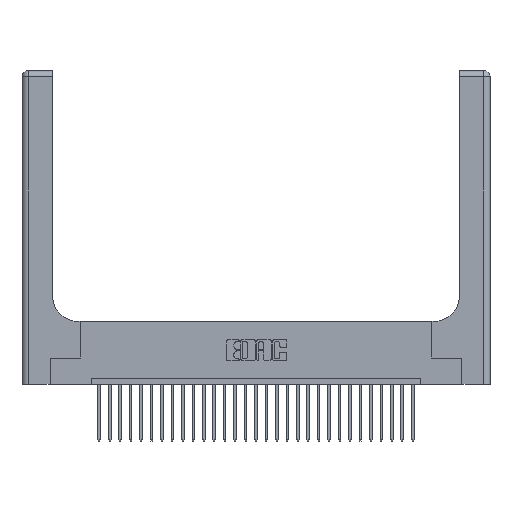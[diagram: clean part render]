
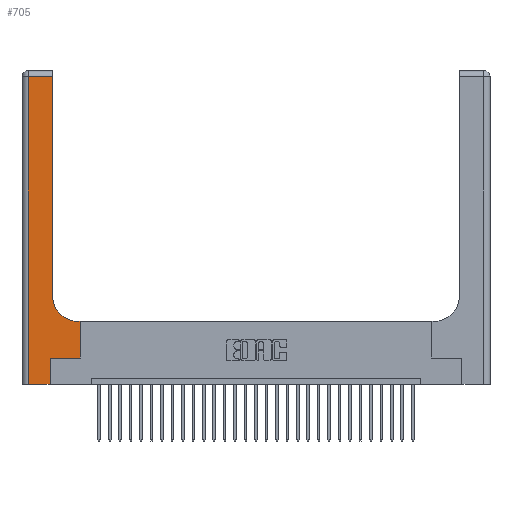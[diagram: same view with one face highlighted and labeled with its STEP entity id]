
A CAD part, top view. The second image highlights one B-rep face of the part: STEP entity #705.
In plain terms, the highlighted planar face has unit normal (0, 0, 1).
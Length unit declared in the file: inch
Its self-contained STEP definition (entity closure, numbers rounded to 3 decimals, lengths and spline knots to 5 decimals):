
#705 = ADVANCED_FACE ( 'NONE', ( #14279 ), #8738, .F. ) ;
#729 = VERTEX_POINT ( 'NONE', #22500 ) ;
#1054 = CARTESIAN_POINT ( 'NONE',  ( 0.2915, 3., 0.37 ) ) ;
#1261 = DIRECTION ( 'NONE',  ( -1., 0., 0. ) ) ;
#1467 = CARTESIAN_POINT ( 'NONE',  ( 0.06, 0., 0.37 ) ) ;
#1710 = DIRECTION ( 'NONE',  ( 0., 1., 0. ) ) ;
#3113 = CARTESIAN_POINT ( 'NONE',  ( 0.5415, 0.6, 0.37 ) ) ;
#3358 = DIRECTION ( 'NONE',  ( 0., 1., 0. ) ) ;
#3384 = ORIENTED_EDGE ( 'NONE', *, *, #9870, .T. ) ;
#3589 = VERTEX_POINT ( 'NONE', #6046 ) ;
#3943 = EDGE_CURVE ( 'NONE', #29154, #3589, #11376, .T. ) ;
#4304 = CARTESIAN_POINT ( 'NONE',  ( 0., 0., 0.37 ) ) ;
#4656 = LINE ( 'NONE', #16124, #25334 ) ;
#4949 = DIRECTION ( 'NONE',  ( 0., -1., 0. ) ) ;
#5971 = LINE ( 'NONE', #13246, #21901 ) ;
#6046 = CARTESIAN_POINT ( 'NONE',  ( 0.2915, 0.85, 0.37 ) ) ;
#6088 = VECTOR ( 'NONE', #1261, 39.37008 ) ;
#6278 = CARTESIAN_POINT ( 'NONE',  ( 0.06, 2.94, 0.37 ) ) ;
#6404 = DIRECTION ( 'NONE',  ( -1., 0., 0. ) ) ;
#7269 = VECTOR ( 'NONE', #21308, 39.37008 ) ;
#7671 = EDGE_CURVE ( 'NONE', #729, #29154, #24580, .T. ) ;
#8009 = LINE ( 'NONE', #14727, #7269 ) ;
#8738 = PLANE ( 'NONE',  #15357 ) ;
#9033 = EDGE_CURVE ( 'NONE', #27274, #27292, #15082, .T. ) ;
#9227 = DIRECTION ( 'NONE',  ( 1., 0., 0. ) ) ;
#9336 = AXIS2_PLACEMENT_3D ( 'NONE', #28037, #25803, #16454 ) ;
#9870 = EDGE_CURVE ( 'NONE', #26841, #729, #5971, .T. ) ;
#9909 = LINE ( 'NONE', #10806, #21162 ) ;
#10383 = EDGE_CURVE ( 'NONE', #23092, #25171, #9909, .T. ) ;
#10715 = ORIENTED_EDGE ( 'NONE', *, *, #24664, .T. ) ;
#10806 = CARTESIAN_POINT ( 'NONE',  ( 0., 2.94, 0.37 ) ) ;
#11376 = CIRCLE ( 'NONE', #9336, 0.25 ) ;
#13116 = LINE ( 'NONE', #1054, #28707 ) ;
#13246 = CARTESIAN_POINT ( 'NONE',  ( 0.5585, 0.25, 0.37 ) ) ;
#13258 = VECTOR ( 'NONE', #27331, 39.37008 ) ;
#13405 = CARTESIAN_POINT ( 'NONE',  ( 0., 3., 0.37 ) ) ;
#14279 = FACE_OUTER_BOUND ( 'NONE', #23038, .T. ) ;
#14501 = VECTOR ( 'NONE', #4949, 39.37008 ) ;
#14727 = CARTESIAN_POINT ( 'NONE',  ( 0.269, 0., 0.37 ) ) ;
#15082 = LINE ( 'NONE', #4304, #13258 ) ;
#15357 = AXIS2_PLACEMENT_3D ( 'NONE', #13405, #22401, #6404 ) ;
#15387 = ORIENTED_EDGE ( 'NONE', *, *, #21820, .T. ) ;
#15731 = ORIENTED_EDGE ( 'NONE', *, *, #23137, .T. ) ;
#16124 = CARTESIAN_POINT ( 'NONE',  ( 0.269, 0.25, 0.37 ) ) ;
#16454 = DIRECTION ( 'NONE',  ( 1., 0., 0. ) ) ;
#17380 = LINE ( 'NONE', #18813, #14501 ) ;
#17891 = DIRECTION ( 'NONE',  ( -1., 0., 0. ) ) ;
#17908 = ORIENTED_EDGE ( 'NONE', *, *, #3943, .T. ) ;
#18813 = CARTESIAN_POINT ( 'NONE',  ( 0.06, 3., 0.37 ) ) ;
#18849 = CARTESIAN_POINT ( 'NONE',  ( 0.2915, 2.94, 0.37 ) ) ;
#18965 = ORIENTED_EDGE ( 'NONE', *, *, #9033, .T. ) ;
#19149 = ORIENTED_EDGE ( 'NONE', *, *, #10383, .T. ) ;
#19775 = CARTESIAN_POINT ( 'NONE',  ( 0.2915, 0.6, 0.37 ) ) ;
#19794 = CARTESIAN_POINT ( 'NONE',  ( 0.269, 0.25, 0.37 ) ) ;
#19985 = EDGE_CURVE ( 'NONE', #27292, #26231, #8009, .T. ) ;
#21162 = VECTOR ( 'NONE', #17891, 39.37008 ) ;
#21308 = DIRECTION ( 'NONE',  ( 0., 1., 0. ) ) ;
#21820 = EDGE_CURVE ( 'NONE', #25171, #27274, #17380, .T. ) ;
#21901 = VECTOR ( 'NONE', #1710, 39.37008 ) ;
#22401 = DIRECTION ( 'NONE',  ( 0., 0., -1. ) ) ;
#22500 = CARTESIAN_POINT ( 'NONE',  ( 0.5585, 0.6, 0.37 ) ) ;
#23038 = EDGE_LOOP ( 'NONE', ( #15731, #19149, #15387, #18965, #27157, #10715, #3384, #26258, #17908 ) ) ;
#23092 = VERTEX_POINT ( 'NONE', #18849 ) ;
#23137 = EDGE_CURVE ( 'NONE', #3589, #23092, #13116, .T. ) ;
#24580 = LINE ( 'NONE', #19775, #6088 ) ;
#24664 = EDGE_CURVE ( 'NONE', #26231, #26841, #4656, .T. ) ;
#25171 = VERTEX_POINT ( 'NONE', #6278 ) ;
#25334 = VECTOR ( 'NONE', #9227, 39.37008 ) ;
#25803 = DIRECTION ( 'NONE',  ( 0., 0., -1. ) ) ;
#26231 = VERTEX_POINT ( 'NONE', #19794 ) ;
#26258 = ORIENTED_EDGE ( 'NONE', *, *, #7671, .T. ) ;
#26841 = VERTEX_POINT ( 'NONE', #27037 ) ;
#27037 = CARTESIAN_POINT ( 'NONE',  ( 0.5585, 0.25, 0.37 ) ) ;
#27157 = ORIENTED_EDGE ( 'NONE', *, *, #19985, .T. ) ;
#27274 = VERTEX_POINT ( 'NONE', #1467 ) ;
#27292 = VERTEX_POINT ( 'NONE', #29819 ) ;
#27331 = DIRECTION ( 'NONE',  ( 1., 0., 0. ) ) ;
#28037 = CARTESIAN_POINT ( 'NONE',  ( 0.5415, 0.85, 0.37 ) ) ;
#28707 = VECTOR ( 'NONE', #3358, 39.37008 ) ;
#29154 = VERTEX_POINT ( 'NONE', #3113 ) ;
#29819 = CARTESIAN_POINT ( 'NONE',  ( 0.269, 0., 0.37 ) ) ;
